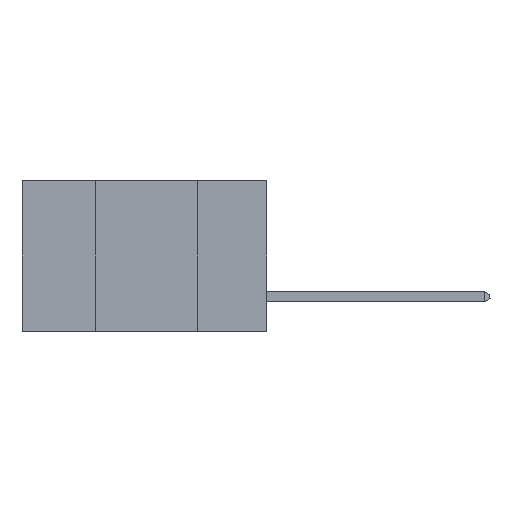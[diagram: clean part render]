
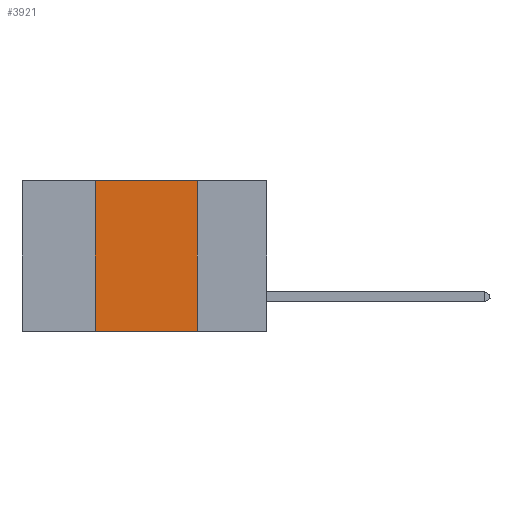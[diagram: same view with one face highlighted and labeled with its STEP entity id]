
A CAD part, left-side view. The second image highlights one B-rep face of the part: STEP entity #3921.
In plain terms, the highlighted planar face has unit normal (-1, 0, 0).
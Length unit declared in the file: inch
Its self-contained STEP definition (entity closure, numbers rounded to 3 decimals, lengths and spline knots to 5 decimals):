
#716 = CARTESIAN_POINT ( 'NONE',  ( 0., 0.6, 0. ) ) ;
#866 = DIRECTION ( 'NONE',  ( 0., -1., 0. ) ) ;
#1730 = ORIENTED_EDGE ( 'NONE', *, *, #11745, .T. ) ;
#1824 = DIRECTION ( 'NONE',  ( 0., 0., -1. ) ) ;
#2019 = CARTESIAN_POINT ( 'NONE',  ( 0., 0.17, -0.37 ) ) ;
#2330 = DIRECTION ( 'NONE',  ( 0., 0., 1. ) ) ;
#2836 = DIRECTION ( 'NONE',  ( 1., 0., 0. ) ) ;
#3180 = LINE ( 'NONE', #7690, #13150 ) ;
#3411 = VERTEX_POINT ( 'NONE', #2019 ) ;
#3856 = DIRECTION ( 'NONE',  ( 0., 0., -1. ) ) ;
#3921 = ADVANCED_FACE ( 'NONE', ( #11242 ), #8181, .F. ) ;
#4842 = CARTESIAN_POINT ( 'NONE',  ( 0., 0.17, 0. ) ) ;
#4943 = LINE ( 'NONE', #13597, #11598 ) ;
#5514 = CARTESIAN_POINT ( 'NONE',  ( 0., 0.42, 0. ) ) ;
#5578 = ORIENTED_EDGE ( 'NONE', *, *, #11359, .F. ) ;
#6769 = VECTOR ( 'NONE', #3856, 39.37008 ) ;
#6821 = CARTESIAN_POINT ( 'NONE',  ( 0., 0.17, 0. ) ) ;
#6839 = AXIS2_PLACEMENT_3D ( 'NONE', #716, #2836, #1824 ) ;
#7690 = CARTESIAN_POINT ( 'NONE',  ( 0., 0.42, 0. ) ) ;
#7897 = DIRECTION ( 'NONE',  ( 0., -1., 0. ) ) ;
#7953 = EDGE_LOOP ( 'NONE', ( #12460, #5578, #9214, #1730 ) ) ;
#8181 = PLANE ( 'NONE',  #6839 ) ;
#8247 = EDGE_CURVE ( 'NONE', #8278, #3411, #12482, .T. ) ;
#8278 = VERTEX_POINT ( 'NONE', #6821 ) ;
#8300 = LINE ( 'NONE', #12158, #10327 ) ;
#9214 = ORIENTED_EDGE ( 'NONE', *, *, #10556, .F. ) ;
#9862 = CARTESIAN_POINT ( 'NONE',  ( 0., 0.42, -0.37 ) ) ;
#10327 = VECTOR ( 'NONE', #7897, 39.37008 ) ;
#10541 = VERTEX_POINT ( 'NONE', #5514 ) ;
#10556 = EDGE_CURVE ( 'NONE', #10940, #10541, #3180, .T. ) ;
#10940 = VERTEX_POINT ( 'NONE', #9862 ) ;
#11242 = FACE_OUTER_BOUND ( 'NONE', #7953, .T. ) ;
#11359 = EDGE_CURVE ( 'NONE', #10541, #8278, #8300, .T. ) ;
#11598 = VECTOR ( 'NONE', #866, 39.37008 ) ;
#11745 = EDGE_CURVE ( 'NONE', #10940, #3411, #4943, .T. ) ;
#12158 = CARTESIAN_POINT ( 'NONE',  ( 0., 0.6, 0. ) ) ;
#12460 = ORIENTED_EDGE ( 'NONE', *, *, #8247, .F. ) ;
#12482 = LINE ( 'NONE', #4842, #6769 ) ;
#13150 = VECTOR ( 'NONE', #2330, 39.37008 ) ;
#13597 = CARTESIAN_POINT ( 'NONE',  ( 0., 0.6, -0.37 ) ) ;
